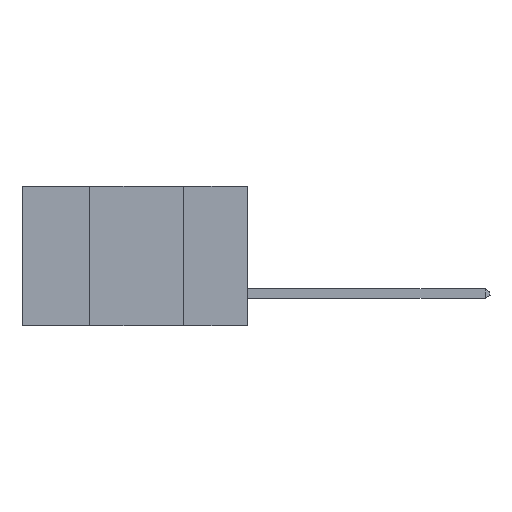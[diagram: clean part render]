
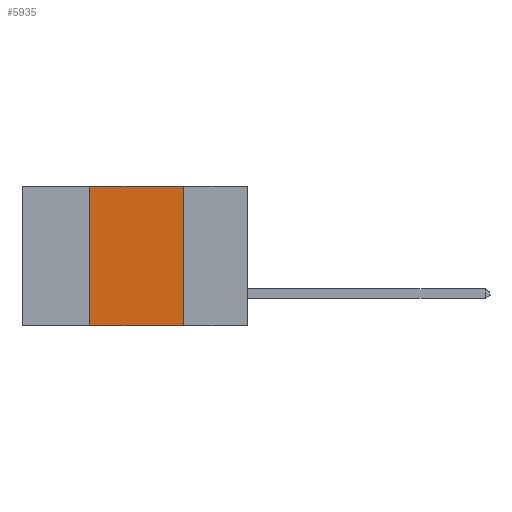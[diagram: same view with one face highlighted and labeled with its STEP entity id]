
A CAD part, left-side view. The second image highlights one B-rep face of the part: STEP entity #5935.
In plain terms, the highlighted planar face has unit normal (-1, 0, 0).
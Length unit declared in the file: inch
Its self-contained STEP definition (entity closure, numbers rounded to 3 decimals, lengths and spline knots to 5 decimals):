
#105 = VERTEX_POINT ( 'NONE', #10738 ) ;
#181 = LINE ( 'NONE', #5238, #9507 ) ;
#380 = PLANE ( 'NONE',  #7622 ) ;
#583 = DIRECTION ( 'NONE',  ( 0., 0., 1. ) ) ;
#682 = CARTESIAN_POINT ( 'NONE',  ( 0., 0.42, -0.37 ) ) ;
#866 = EDGE_CURVE ( 'NONE', #105, #9796, #1357, .T. ) ;
#1357 = LINE ( 'NONE', #5680, #2029 ) ;
#1386 = EDGE_LOOP ( 'NONE', ( #10751, #10926, #5647, #3391 ) ) ;
#2029 = VECTOR ( 'NONE', #6699, 39.37008 ) ;
#2208 = CARTESIAN_POINT ( 'NONE',  ( 0., 0.6, 0. ) ) ;
#3391 = ORIENTED_EDGE ( 'NONE', *, *, #7988, .T. ) ;
#3682 = FACE_OUTER_BOUND ( 'NONE', #1386, .T. ) ;
#3710 = EDGE_CURVE ( 'NONE', #7069, #105, #181, .T. ) ;
#3912 = DIRECTION ( 'NONE',  ( 0., 0., -1. ) ) ;
#5080 = VECTOR ( 'NONE', #583, 39.37008 ) ;
#5238 = CARTESIAN_POINT ( 'NONE',  ( 0., 0.6, 0. ) ) ;
#5647 = ORIENTED_EDGE ( 'NONE', *, *, #6904, .F. ) ;
#5680 = CARTESIAN_POINT ( 'NONE',  ( 0., 0.17, 0. ) ) ;
#5935 = ADVANCED_FACE ( 'NONE', ( #3682 ), #380, .F. ) ;
#6328 = VECTOR ( 'NONE', #8329, 39.37008 ) ;
#6358 = VERTEX_POINT ( 'NONE', #682 ) ;
#6688 = DIRECTION ( 'NONE',  ( 1., 0., 0. ) ) ;
#6699 = DIRECTION ( 'NONE',  ( 0., 0., -1. ) ) ;
#6904 = EDGE_CURVE ( 'NONE', #6358, #7069, #10851, .T. ) ;
#6973 = CARTESIAN_POINT ( 'NONE',  ( 0., 0.42, 0. ) ) ;
#7069 = VERTEX_POINT ( 'NONE', #7246 ) ;
#7246 = CARTESIAN_POINT ( 'NONE',  ( 0., 0.42, 0. ) ) ;
#7622 = AXIS2_PLACEMENT_3D ( 'NONE', #2208, #6688, #3912 ) ;
#7988 = EDGE_CURVE ( 'NONE', #6358, #9796, #8302, .T. ) ;
#8302 = LINE ( 'NONE', #10112, #6328 ) ;
#8329 = DIRECTION ( 'NONE',  ( 0., -1., 0. ) ) ;
#9275 = CARTESIAN_POINT ( 'NONE',  ( 0., 0.17, -0.37 ) ) ;
#9507 = VECTOR ( 'NONE', #9713, 39.37008 ) ;
#9713 = DIRECTION ( 'NONE',  ( 0., -1., 0. ) ) ;
#9796 = VERTEX_POINT ( 'NONE', #9275 ) ;
#10112 = CARTESIAN_POINT ( 'NONE',  ( 0., 0.6, -0.37 ) ) ;
#10738 = CARTESIAN_POINT ( 'NONE',  ( 0., 0.17, 0. ) ) ;
#10751 = ORIENTED_EDGE ( 'NONE', *, *, #866, .F. ) ;
#10851 = LINE ( 'NONE', #6973, #5080 ) ;
#10926 = ORIENTED_EDGE ( 'NONE', *, *, #3710, .F. ) ;
